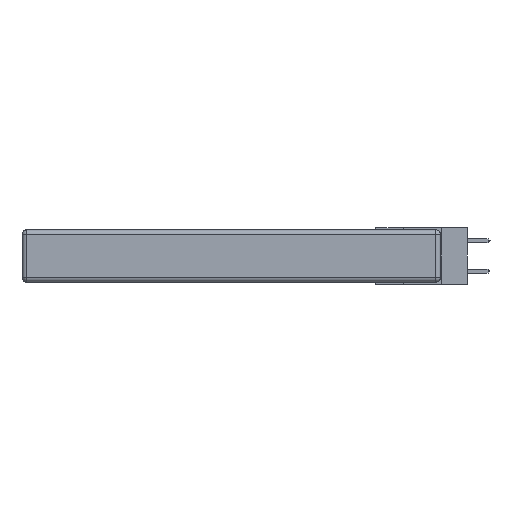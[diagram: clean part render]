
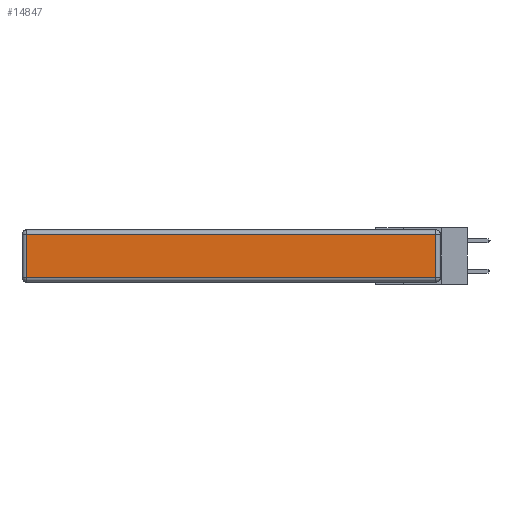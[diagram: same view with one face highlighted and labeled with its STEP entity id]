
A CAD part, left-side view. The second image highlights one B-rep face of the part: STEP entity #14847.
In plain terms, the highlighted planar face has unit normal (-1, 0, 0).
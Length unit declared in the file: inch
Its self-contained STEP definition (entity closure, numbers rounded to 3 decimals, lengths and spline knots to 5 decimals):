
#130 = VECTOR ( 'NONE', #367, 39.37008 ) ;
#367 = DIRECTION ( 'NONE',  ( 0., 1., 0. ) ) ;
#891 = DIRECTION ( 'NONE',  ( 0., -1., 0. ) ) ;
#3010 = DIRECTION ( 'NONE',  ( 0., 0., 1. ) ) ;
#6408 = DIRECTION ( 'NONE',  ( 0., 0., -1. ) ) ;
#7096 = CARTESIAN_POINT ( 'NONE',  ( 0., 0., -0.313 ) ) ;
#7645 = VERTEX_POINT ( 'NONE', #25001 ) ;
#8216 = CARTESIAN_POINT ( 'NONE',  ( 0., 0.03, -0.313 ) ) ;
#8266 = CARTESIAN_POINT ( 'NONE',  ( 0., 2.75, -0.03 ) ) ;
#8563 = CARTESIAN_POINT ( 'NONE',  ( 0., 2.72, -0.313 ) ) ;
#9382 = VECTOR ( 'NONE', #891, 39.37008 ) ;
#10127 = CARTESIAN_POINT ( 'NONE',  ( 0., 0., -0.343 ) ) ;
#10218 = VERTEX_POINT ( 'NONE', #10793 ) ;
#10265 = CARTESIAN_POINT ( 'NONE',  ( 0., 2.72, -0.343 ) ) ;
#10793 = CARTESIAN_POINT ( 'NONE',  ( 0., 0.03, -0.03 ) ) ;
#11942 = LINE ( 'NONE', #7096, #9382 ) ;
#12143 = EDGE_CURVE ( 'NONE', #10218, #7645, #17749, .T. ) ;
#12318 = VERTEX_POINT ( 'NONE', #8216 ) ;
#12447 = LINE ( 'NONE', #25269, #17225 ) ;
#13188 = EDGE_CURVE ( 'NONE', #7645, #18997, #23465, .T. ) ;
#14847 = ADVANCED_FACE ( 'NONE', ( #15997 ), #20300, .T. ) ;
#15997 = FACE_OUTER_BOUND ( 'NONE', #17662, .T. ) ;
#17225 = VECTOR ( 'NONE', #3010, 39.37008 ) ;
#17662 = EDGE_LOOP ( 'NONE', ( #24107, #21011, #23811, #18831 ) ) ;
#17749 = LINE ( 'NONE', #8266, #130 ) ;
#18323 = EDGE_CURVE ( 'NONE', #18997, #12318, #11942, .T. ) ;
#18831 = ORIENTED_EDGE ( 'NONE', *, *, #13188, .T. ) ;
#18997 = VERTEX_POINT ( 'NONE', #8563 ) ;
#19304 = VECTOR ( 'NONE', #6408, 39.37008 ) ;
#20115 = DIRECTION ( 'NONE',  ( -1., 0., 0. ) ) ;
#20205 = DIRECTION ( 'NONE',  ( 0., 0., 1. ) ) ;
#20300 = PLANE ( 'NONE',  #22263 ) ;
#21011 = ORIENTED_EDGE ( 'NONE', *, *, #26077, .T. ) ;
#22263 = AXIS2_PLACEMENT_3D ( 'NONE', #10127, #20115, #20205 ) ;
#23465 = LINE ( 'NONE', #10265, #19304 ) ;
#23811 = ORIENTED_EDGE ( 'NONE', *, *, #12143, .T. ) ;
#24107 = ORIENTED_EDGE ( 'NONE', *, *, #18323, .T. ) ;
#25001 = CARTESIAN_POINT ( 'NONE',  ( 0., 2.72, -0.03 ) ) ;
#25269 = CARTESIAN_POINT ( 'NONE',  ( 0., 0.03, -0.343 ) ) ;
#26077 = EDGE_CURVE ( 'NONE', #12318, #10218, #12447, .T. ) ;
